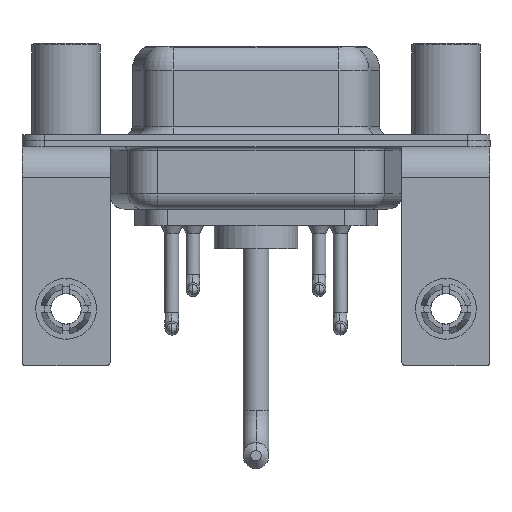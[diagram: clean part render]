
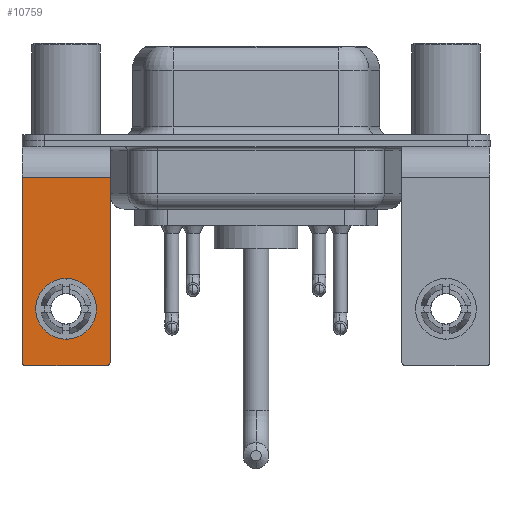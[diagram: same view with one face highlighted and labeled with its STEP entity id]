
A CAD part, front view. The second image highlights one B-rep face of the part: STEP entity #10759.
In plain terms, the highlighted planar face has unit normal (0, -1, 0).
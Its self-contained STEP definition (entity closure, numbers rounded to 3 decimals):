
#24 = DIRECTION ( 'NONE',  ( 0., 0., 1. ) ) ;
#33 = CARTESIAN_POINT ( 'NONE',  ( -2.9, -6.25, -2.4 ) ) ;
#91 = EDGE_CURVE ( 'NONE', #13000, #5607, #17599, .T. ) ;
#96 = CARTESIAN_POINT ( 'NONE',  ( 2.9, -6.25, -2.4 ) ) ;
#134 = ORIENTED_EDGE ( 'NONE', *, *, #412, .T. ) ;
#287 = DIRECTION ( 'NONE',  ( 0., 1., 0. ) ) ;
#412 = EDGE_CURVE ( 'NONE', #12715, #18378, #12743, .T. ) ;
#437 = VERTEX_POINT ( 'NONE', #16360 ) ;
#799 = ORIENTED_EDGE ( 'NONE', *, *, #3835, .T. ) ;
#1220 = CARTESIAN_POINT ( 'NONE',  ( -2.9, -6.25, -14.55 ) ) ;
#1795 = FACE_OUTER_BOUND ( 'NONE', #19062, .T. ) ;
#1879 = EDGE_CURVE ( 'NONE', #2365, #10994, #5393, .T. ) ;
#2259 = AXIS2_PLACEMENT_3D ( 'NONE', #3937, #10060, #16162 ) ;
#2365 = VERTEX_POINT ( 'NONE', #1220 ) ;
#3438 = CARTESIAN_POINT ( 'NONE',  ( 2.9, -6.25, -14.8 ) ) ;
#3554 = CIRCLE ( 'NONE', #14759, 2. ) ;
#3735 = AXIS2_PLACEMENT_3D ( 'NONE', #96, #287, #6406 ) ;
#3787 = CARTESIAN_POINT ( 'NONE',  ( 0., -6.25, -9.07 ) ) ;
#3835 = EDGE_CURVE ( 'NONE', #5607, #2365, #13961, .T. ) ;
#3937 = CARTESIAN_POINT ( 'NONE',  ( 0., -6.25, -11.07 ) ) ;
#4101 = AXIS2_PLACEMENT_3D ( 'NONE', #10443, #11757, #8736 ) ;
#4154 = EDGE_CURVE ( 'NONE', #13809, #437, #13143, .T. ) ;
#4181 = ORIENTED_EDGE ( 'NONE', *, *, #17063, .T. ) ;
#4392 = ORIENTED_EDGE ( 'NONE', *, *, #1879, .T. ) ;
#4537 = PLANE ( 'NONE',  #3735 ) ;
#4557 = DIRECTION ( 'NONE',  ( 0., 0., -1. ) ) ;
#4870 = ORIENTED_EDGE ( 'NONE', *, *, #91, .T. ) ;
#5046 = LINE ( 'NONE', #3438, #18350 ) ;
#5393 = CIRCLE ( 'NONE', #6978, 0.25 ) ;
#5607 = VERTEX_POINT ( 'NONE', #33 ) ;
#5657 = LINE ( 'NONE', #5853, #15115 ) ;
#5853 = CARTESIAN_POINT ( 'NONE',  ( 2.9, -6.25, -2.4 ) ) ;
#5861 = EDGE_CURVE ( 'NONE', #13000, #18378, #5657, .T. ) ;
#6406 = DIRECTION ( 'NONE',  ( 0., 0., 1. ) ) ;
#6541 = CARTESIAN_POINT ( 'NONE',  ( 2.9, -6.25, -14.55 ) ) ;
#6620 = CARTESIAN_POINT ( 'NONE',  ( 2.9, -6.25, -2.4 ) ) ;
#6859 = DIRECTION ( 'NONE',  ( -1., 0., 0. ) ) ;
#6978 = AXIS2_PLACEMENT_3D ( 'NONE', #13200, #17913, #19328 ) ;
#7237 = CARTESIAN_POINT ( 'NONE',  ( 2.65, -6.25, -14.8 ) ) ;
#7643 = CARTESIAN_POINT ( 'NONE',  ( 0., -6.25, -11.07 ) ) ;
#8248 = VECTOR ( 'NONE', #6859, 1000. ) ;
#8729 = EDGE_CURVE ( 'NONE', #12715, #10994, #5046, .T. ) ;
#8736 = DIRECTION ( 'NONE',  ( 0., 0., 1. ) ) ;
#9880 = CARTESIAN_POINT ( 'NONE',  ( 2.9, -6.25, -2.4 ) ) ;
#10060 = DIRECTION ( 'NONE',  ( 0., 1., 0. ) ) ;
#10443 = CARTESIAN_POINT ( 'NONE',  ( 2.65, -6.25, -14.55 ) ) ;
#10759 = ADVANCED_FACE ( 'NONE', ( #15447, #1795 ), #4537, .F. ) ;
#10994 = VERTEX_POINT ( 'NONE', #14092 ) ;
#11757 = DIRECTION ( 'NONE',  ( 0., -1., 0. ) ) ;
#12390 = ORIENTED_EDGE ( 'NONE', *, *, #8729, .F. ) ;
#12715 = VERTEX_POINT ( 'NONE', #7237 ) ;
#12743 = CIRCLE ( 'NONE', #4101, 0.25 ) ;
#12860 = ORIENTED_EDGE ( 'NONE', *, *, #5861, .F. ) ;
#13000 = VERTEX_POINT ( 'NONE', #6620 ) ;
#13143 = CIRCLE ( 'NONE', #2259, 2. ) ;
#13200 = CARTESIAN_POINT ( 'NONE',  ( -2.65, -6.25, -14.55 ) ) ;
#13783 = DIRECTION ( 'NONE',  ( 0., 1., 0. ) ) ;
#13809 = VERTEX_POINT ( 'NONE', #3787 ) ;
#13961 = LINE ( 'NONE', #18288, #19549 ) ;
#14092 = CARTESIAN_POINT ( 'NONE',  ( -2.65, -6.25, -14.8 ) ) ;
#14519 = EDGE_LOOP ( 'NONE', ( #4181, #18107 ) ) ;
#14759 = AXIS2_PLACEMENT_3D ( 'NONE', #7643, #13783, #24 ) ;
#15115 = VECTOR ( 'NONE', #18089, 1000. ) ;
#15447 = FACE_BOUND ( 'NONE', #14519, .T. ) ;
#15667 = DIRECTION ( 'NONE',  ( -1., 0., 0. ) ) ;
#16162 = DIRECTION ( 'NONE',  ( 0., 0., 1. ) ) ;
#16360 = CARTESIAN_POINT ( 'NONE',  ( 0., -6.25, -13.07 ) ) ;
#17063 = EDGE_CURVE ( 'NONE', #437, #13809, #3554, .T. ) ;
#17599 = LINE ( 'NONE', #9880, #8248 ) ;
#17913 = DIRECTION ( 'NONE',  ( 0., -1., 0. ) ) ;
#18089 = DIRECTION ( 'NONE',  ( 0., 0., -1. ) ) ;
#18107 = ORIENTED_EDGE ( 'NONE', *, *, #4154, .T. ) ;
#18288 = CARTESIAN_POINT ( 'NONE',  ( -2.9, -6.25, -2.4 ) ) ;
#18350 = VECTOR ( 'NONE', #15667, 1000. ) ;
#18378 = VERTEX_POINT ( 'NONE', #6541 ) ;
#19062 = EDGE_LOOP ( 'NONE', ( #799, #4392, #12390, #134, #12860, #4870 ) ) ;
#19328 = DIRECTION ( 'NONE',  ( 0., 0., 1. ) ) ;
#19549 = VECTOR ( 'NONE', #4557, 1000. ) ;
